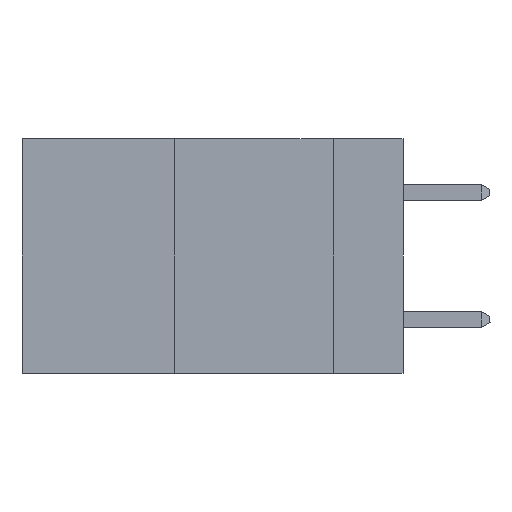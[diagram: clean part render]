
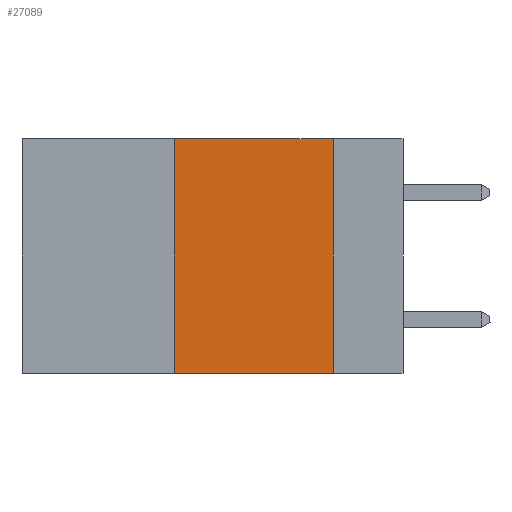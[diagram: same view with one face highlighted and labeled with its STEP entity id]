
A CAD part, left-side view. The second image highlights one B-rep face of the part: STEP entity #27089.
In plain terms, the highlighted planar face has unit normal (-1, 0, 0).
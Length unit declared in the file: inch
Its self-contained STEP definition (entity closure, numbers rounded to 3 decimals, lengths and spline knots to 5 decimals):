
#157 = LINE ( 'NONE', #21467, #10450 ) ;
#1492 = FACE_OUTER_BOUND ( 'NONE', #10996, .T. ) ;
#1967 = VERTEX_POINT ( 'NONE', #8579 ) ;
#3189 = VECTOR ( 'NONE', #20825, 39.37008 ) ;
#3752 = CARTESIAN_POINT ( 'NONE',  ( 0., 0.11, 0. ) ) ;
#4979 = CARTESIAN_POINT ( 'NONE',  ( 0., 0.11, -0.37 ) ) ;
#6541 = CARTESIAN_POINT ( 'NONE',  ( 0., 0.11, 0. ) ) ;
#6624 = ORIENTED_EDGE ( 'NONE', *, *, #16153, .F. ) ;
#8579 = CARTESIAN_POINT ( 'NONE',  ( 0., 0.36, -0.37 ) ) ;
#8591 = CARTESIAN_POINT ( 'NONE',  ( 0., 0.6, -0.37 ) ) ;
#8671 = EDGE_CURVE ( 'NONE', #1967, #19707, #19610, .T. ) ;
#8735 = DIRECTION ( 'NONE',  ( 0., -1., 0. ) ) ;
#10450 = VECTOR ( 'NONE', #25940, 39.37008 ) ;
#10796 = AXIS2_PLACEMENT_3D ( 'NONE', #18608, #20146, #25032 ) ;
#10996 = EDGE_LOOP ( 'NONE', ( #6624, #18138, #27123, #24058 ) ) ;
#11287 = VECTOR ( 'NONE', #15344, 39.37008 ) ;
#13102 = CARTESIAN_POINT ( 'NONE',  ( 0., 0.6, 0. ) ) ;
#15344 = DIRECTION ( 'NONE',  ( 0., -1., 0. ) ) ;
#16153 = EDGE_CURVE ( 'NONE', #16706, #19707, #23064, .T. ) ;
#16674 = EDGE_CURVE ( 'NONE', #20717, #16706, #23448, .T. ) ;
#16706 = VERTEX_POINT ( 'NONE', #6541 ) ;
#18138 = ORIENTED_EDGE ( 'NONE', *, *, #16674, .F. ) ;
#18589 = EDGE_CURVE ( 'NONE', #1967, #20717, #157, .T. ) ;
#18608 = CARTESIAN_POINT ( 'NONE',  ( 0., 0.6, 0. ) ) ;
#19610 = LINE ( 'NONE', #8591, #27292 ) ;
#19707 = VERTEX_POINT ( 'NONE', #4979 ) ;
#20146 = DIRECTION ( 'NONE',  ( 1., 0., 0. ) ) ;
#20416 = PLANE ( 'NONE',  #10796 ) ;
#20717 = VERTEX_POINT ( 'NONE', #24469 ) ;
#20825 = DIRECTION ( 'NONE',  ( 0., 0., -1. ) ) ;
#21467 = CARTESIAN_POINT ( 'NONE',  ( 0., 0.36, 0. ) ) ;
#23064 = LINE ( 'NONE', #3752, #3189 ) ;
#23448 = LINE ( 'NONE', #13102, #11287 ) ;
#24058 = ORIENTED_EDGE ( 'NONE', *, *, #8671, .T. ) ;
#24469 = CARTESIAN_POINT ( 'NONE',  ( 0., 0.36, 0. ) ) ;
#25032 = DIRECTION ( 'NONE',  ( 0., 0., -1. ) ) ;
#25940 = DIRECTION ( 'NONE',  ( 0., 0., 1. ) ) ;
#27089 = ADVANCED_FACE ( 'NONE', ( #1492 ), #20416, .F. ) ;
#27123 = ORIENTED_EDGE ( 'NONE', *, *, #18589, .F. ) ;
#27292 = VECTOR ( 'NONE', #8735, 39.37008 ) ;
